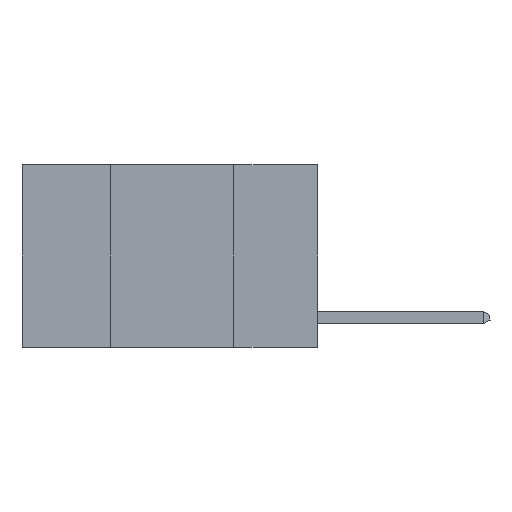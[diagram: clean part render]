
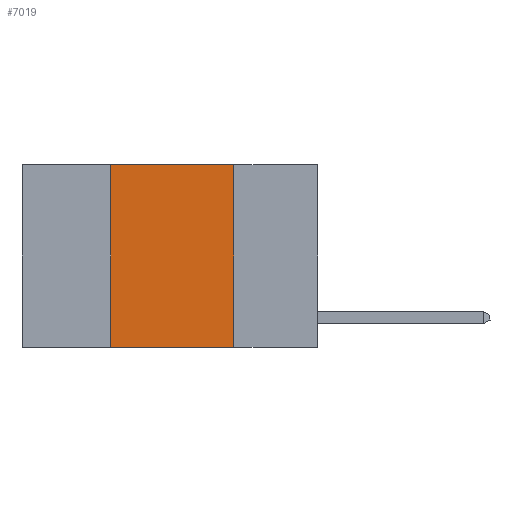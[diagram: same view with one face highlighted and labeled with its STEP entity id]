
A CAD part, left-side view. The second image highlights one B-rep face of the part: STEP entity #7019.
In plain terms, the highlighted planar face has unit normal (-1, 0, 0).
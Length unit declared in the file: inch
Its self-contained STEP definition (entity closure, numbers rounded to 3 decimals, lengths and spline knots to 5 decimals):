
#63 = DIRECTION ( 'NONE',  ( 0., 0., -1. ) ) ;
#587 = ORIENTED_EDGE ( 'NONE', *, *, #4057, .F. ) ;
#634 = EDGE_CURVE ( 'NONE', #1184, #10155, #8395, .T. ) ;
#1001 = VECTOR ( 'NONE', #7922, 39.37008 ) ;
#1184 = VERTEX_POINT ( 'NONE', #8402 ) ;
#1310 = VERTEX_POINT ( 'NONE', #6242 ) ;
#1400 = VECTOR ( 'NONE', #1515, 39.37008 ) ;
#1515 = DIRECTION ( 'NONE',  ( 0., -1., 0. ) ) ;
#2569 = CARTESIAN_POINT ( 'NONE',  ( 0., 0.6, 0. ) ) ;
#2825 = ORIENTED_EDGE ( 'NONE', *, *, #9233, .F. ) ;
#2888 = EDGE_CURVE ( 'NONE', #1184, #6079, #5497, .T. ) ;
#3747 = EDGE_LOOP ( 'NONE', ( #587, #2825, #7342, #9581 ) ) ;
#3861 = DIRECTION ( 'NONE',  ( 0., -1., 0. ) ) ;
#3989 = CARTESIAN_POINT ( 'NONE',  ( 0., 0.6, -0.37 ) ) ;
#4057 = EDGE_CURVE ( 'NONE', #1310, #10155, #10451, .T. ) ;
#4333 = DIRECTION ( 'NONE',  ( 0., 0., -1. ) ) ;
#5143 = PLANE ( 'NONE',  #8164 ) ;
#5497 = LINE ( 'NONE', #7065, #1001 ) ;
#6079 = VERTEX_POINT ( 'NONE', #9877 ) ;
#6174 = VECTOR ( 'NONE', #3861, 39.37008 ) ;
#6242 = CARTESIAN_POINT ( 'NONE',  ( 0., 0.17, 0. ) ) ;
#7019 = ADVANCED_FACE ( 'NONE', ( #8030 ), #5143, .F. ) ;
#7065 = CARTESIAN_POINT ( 'NONE',  ( 0., 0.42, 0. ) ) ;
#7342 = ORIENTED_EDGE ( 'NONE', *, *, #2888, .F. ) ;
#7431 = CARTESIAN_POINT ( 'NONE',  ( 0., 0.6, 0. ) ) ;
#7922 = DIRECTION ( 'NONE',  ( 0., 0., 1. ) ) ;
#8030 = FACE_OUTER_BOUND ( 'NONE', #3747, .T. ) ;
#8132 = LINE ( 'NONE', #7431, #1400 ) ;
#8164 = AXIS2_PLACEMENT_3D ( 'NONE', #2569, #9359, #4333 ) ;
#8232 = VECTOR ( 'NONE', #63, 39.37008 ) ;
#8395 = LINE ( 'NONE', #3989, #6174 ) ;
#8402 = CARTESIAN_POINT ( 'NONE',  ( 0., 0.42, -0.37 ) ) ;
#8724 = CARTESIAN_POINT ( 'NONE',  ( 0., 0.17, -0.37 ) ) ;
#9233 = EDGE_CURVE ( 'NONE', #6079, #1310, #8132, .T. ) ;
#9348 = CARTESIAN_POINT ( 'NONE',  ( 0., 0.17, 0. ) ) ;
#9359 = DIRECTION ( 'NONE',  ( 1., 0., 0. ) ) ;
#9581 = ORIENTED_EDGE ( 'NONE', *, *, #634, .T. ) ;
#9877 = CARTESIAN_POINT ( 'NONE',  ( 0., 0.42, 0. ) ) ;
#10155 = VERTEX_POINT ( 'NONE', #8724 ) ;
#10451 = LINE ( 'NONE', #9348, #8232 ) ;
